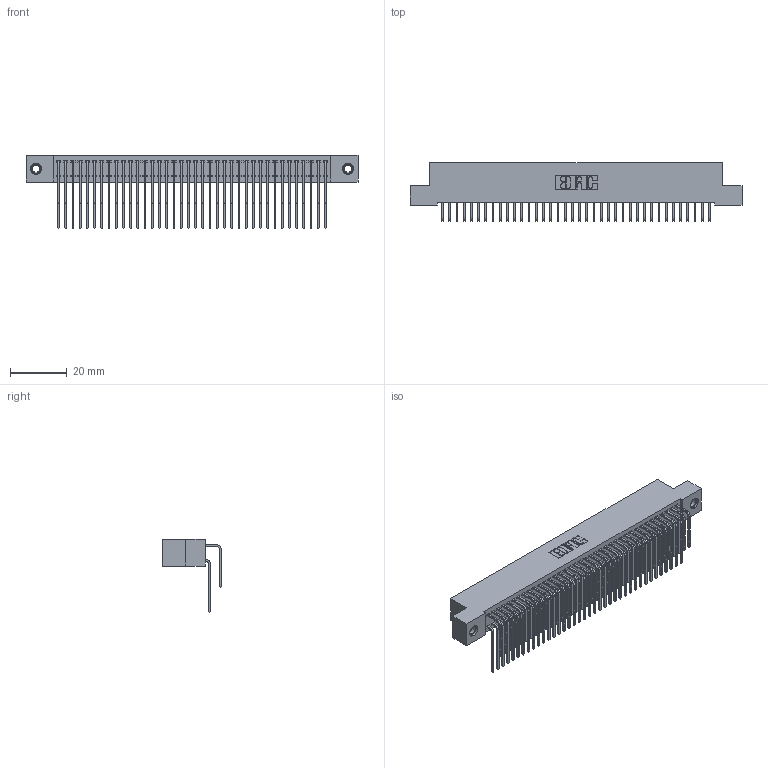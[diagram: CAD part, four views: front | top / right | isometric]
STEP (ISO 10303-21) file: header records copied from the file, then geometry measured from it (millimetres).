
FILE_DESCRIPTION (( 'STEP AP203' ), '1' );
FILE_NAME ('342-076-559-207.STEP', '2019-10-04T10:56:32', ( '' ), ( '' ), 'SwSTEP 2.0', 'SolidWorks 2016', '' );
FILE_SCHEMA (( 'CONFIG_CONTROL_DESIGN' ));
Length unit declared in the file: inch
Products named in the file (5): 345-292-001_559 Tail - 2; 345-250-001_345-250-005-103; 342-076-559-207; 342 Part_TI; 345-292-001_558 559 Tail - 1
Assembly tree (79 placements, depth 2):
  342-076-559-207
    342 Part_TI
    345-292-001_558 559 Tail - 1  x38
    345-292-001_559 Tail - 2  x38
    345-250-001_345-250-005-103  x2
Bounding box: 116.84 x 20.64 x 25.78 mm (x, y, z)
Volume: 10904.9 mm3; surface area: 19660.9 mm2
Topology: 79 solids, 79 shells, 4274 faces, 12671 edges, 8338 vertices
Faces by surface type: plane 2986, cylinder 1272, cone 12, torus 4
Entity records: 27802 total; most frequent: CARTESIAN_POINT 4644, ORIENTED_EDGE 4522, DIRECTION 3987, EDGE_CURVE 2261, LINE 2073, VECTOR 2073, VERTEX_POINT 1500, AXIS2_PLACEMENT_3D 957
